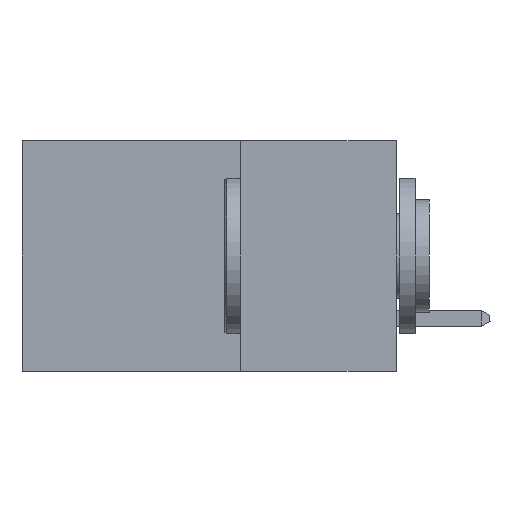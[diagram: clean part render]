
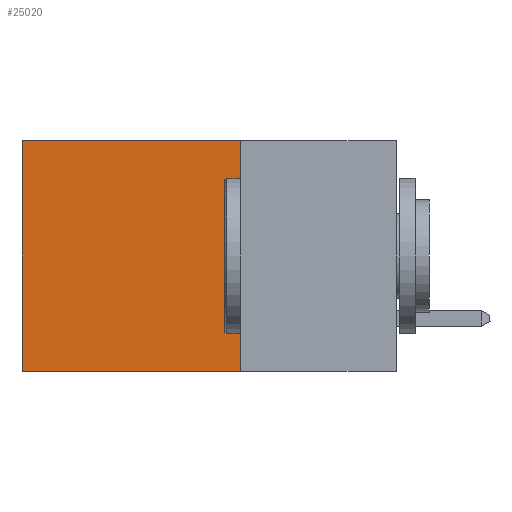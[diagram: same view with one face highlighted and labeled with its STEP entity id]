
A CAD part, left-side view. The second image highlights one B-rep face of the part: STEP entity #25020.
In plain terms, the highlighted planar face has unit normal (-1, 0, 0).
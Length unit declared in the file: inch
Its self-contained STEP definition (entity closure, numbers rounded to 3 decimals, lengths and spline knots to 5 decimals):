
#876 = VECTOR ( 'NONE', #23568, 39.37008 ) ;
#1039 = CARTESIAN_POINT ( 'NONE',  ( 0.298, 0.25, -0.37 ) ) ;
#3658 = ORIENTED_EDGE ( 'NONE', *, *, #6131, .T. ) ;
#5376 = PLANE ( 'NONE',  #15862 ) ;
#6131 = EDGE_CURVE ( 'NONE', #25347, #24157, #9550, .T. ) ;
#7055 = EDGE_CURVE ( 'NONE', #25347, #25562, #14211, .T. ) ;
#7387 = DIRECTION ( 'NONE',  ( 0., 1., 0. ) ) ;
#7693 = DIRECTION ( 'NONE',  ( 0., 0., -1. ) ) ;
#9550 = LINE ( 'NONE', #12454, #876 ) ;
#9826 = CARTESIAN_POINT ( 'NONE',  ( 0.298, 0.25, 0. ) ) ;
#10320 = DIRECTION ( 'NONE',  ( 0., 0., -1. ) ) ;
#11477 = CARTESIAN_POINT ( 'NONE',  ( 0.298, 0.6, 0. ) ) ;
#12454 = CARTESIAN_POINT ( 'NONE',  ( 0.298, 0.25, 0. ) ) ;
#12683 = CARTESIAN_POINT ( 'NONE',  ( 0.298, 0.25, 0. ) ) ;
#12931 = LINE ( 'NONE', #14278, #23396 ) ;
#14211 = LINE ( 'NONE', #12683, #18751 ) ;
#14278 = CARTESIAN_POINT ( 'NONE',  ( 0.298, 0.25, -0.37 ) ) ;
#14764 = LINE ( 'NONE', #24873, #19337 ) ;
#15765 = EDGE_CURVE ( 'NONE', #24157, #18061, #14764, .T. ) ;
#15862 = AXIS2_PLACEMENT_3D ( 'NONE', #9826, #21018, #7693 ) ;
#16138 = CARTESIAN_POINT ( 'NONE',  ( 0.298, 0.6, -0.37 ) ) ;
#17965 = DIRECTION ( 'NONE',  ( 0., 0., -1. ) ) ;
#18061 = VERTEX_POINT ( 'NONE', #16138 ) ;
#18310 = EDGE_CURVE ( 'NONE', #25562, #18061, #12931, .T. ) ;
#18362 = ORIENTED_EDGE ( 'NONE', *, *, #7055, .F. ) ;
#18751 = VECTOR ( 'NONE', #10320, 39.37008 ) ;
#19337 = VECTOR ( 'NONE', #17965, 39.37008 ) ;
#19518 = EDGE_LOOP ( 'NONE', ( #24824, #28653, #18362, #3658 ) ) ;
#21018 = DIRECTION ( 'NONE',  ( 1., 0., 0. ) ) ;
#23396 = VECTOR ( 'NONE', #7387, 39.37008 ) ;
#23568 = DIRECTION ( 'NONE',  ( 0., 1., 0. ) ) ;
#24157 = VERTEX_POINT ( 'NONE', #11477 ) ;
#24286 = FACE_OUTER_BOUND ( 'NONE', #19518, .T. ) ;
#24824 = ORIENTED_EDGE ( 'NONE', *, *, #15765, .T. ) ;
#24873 = CARTESIAN_POINT ( 'NONE',  ( 0.298, 0.6, 0. ) ) ;
#25020 = ADVANCED_FACE ( 'NONE', ( #24286 ), #5376, .F. ) ;
#25347 = VERTEX_POINT ( 'NONE', #26451 ) ;
#25562 = VERTEX_POINT ( 'NONE', #1039 ) ;
#26451 = CARTESIAN_POINT ( 'NONE',  ( 0.298, 0.25, 0. ) ) ;
#28653 = ORIENTED_EDGE ( 'NONE', *, *, #18310, .F. ) ;
